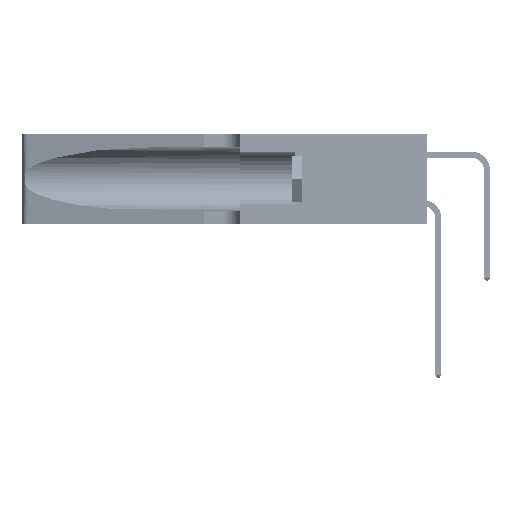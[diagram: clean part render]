
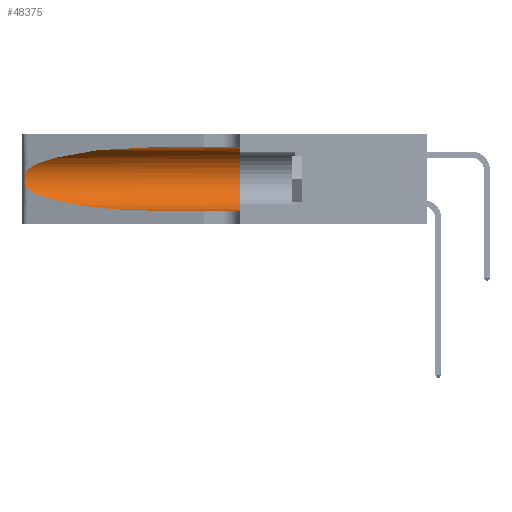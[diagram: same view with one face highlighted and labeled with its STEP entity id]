
A CAD part, left-side view. The second image highlights one B-rep face of the part: STEP entity #48375.
In plain terms, the highlighted cylindrical face has radius 3.308 mm (diameter 6.617 mm), a partial arc.
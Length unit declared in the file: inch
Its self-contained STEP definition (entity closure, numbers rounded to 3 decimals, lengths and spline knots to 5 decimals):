
#54 = ORIENTED_EDGE ( 'NONE', *, *, #10512, .F. ) ;
#1096 = DIRECTION ( 'NONE',  ( 0., 0., 1. ) ) ;
#1575 = CYLINDRICAL_SURFACE ( 'NONE', #9185, 0.13025 ) ;
#2774 = FACE_OUTER_BOUND ( 'NONE', #11011, .T. ) ;
#3232 = DIRECTION ( 'NONE',  ( 0., 0., -1. ) ) ;
#3896 = EDGE_CURVE ( 'NONE', #20273, #45783, #6165, .T. ) ;
#4743 = CARTESIAN_POINT ( 'NONE',  ( 0.25487, 1.22718, 0.14631 ) ) ;
#5531 = VERTEX_POINT ( 'NONE', #31249 ) ;
#5958 = CARTESIAN_POINT ( 'NONE',  ( 0.25787, 1.23484, 0.2124 ) ) ;
#6165 = LINE ( 'NONE', #10392, #45437 ) ;
#8508 = CARTESIAN_POINT ( 'NONE',  ( 0.25487, 1.22718, 0.22369 ) ) ;
#8658 = CARTESIAN_POINT ( 'NONE',  ( 0.2373, 1.15595, 0.08982 ) ) ;
#9185 = AXIS2_PLACEMENT_3D ( 'NONE', #18717, #41415, #3232 ) ;
#9362 = EDGE_CURVE ( 'NONE', #5531, #28183, #43815, .T. ) ;
#9848 = CARTESIAN_POINT ( 'NONE',  ( 0.26018, 1.23835, 0.19895 ) ) ;
#10392 = CARTESIAN_POINT ( 'NONE',  ( 0.1305, 1.61858, 0.05475 ) ) ;
#10512 = EDGE_CURVE ( 'NONE', #43008, #35788, #24158, .T. ) ;
#11011 = EDGE_LOOP ( 'NONE', ( #44678, #37558, #48552, #19919, #36884, #54 ) ) ;
#12550 = CARTESIAN_POINT ( 'NONE',  ( 0.1305, 0.72297, 0.05475 ) ) ;
#12875 = VECTOR ( 'NONE', #21083, 39.37008 ) ;
#13599 = CARTESIAN_POINT ( 'NONE',  ( 0.1305, 1.61858, 0.31525 ) ) ;
#13711 = CARTESIAN_POINT ( 'NONE',  ( 0.26075, 1.23896, 0.178 ) ) ;
#15723 = CIRCLE ( 'NONE', #29706, 0.13025 ) ;
#17556 = CARTESIAN_POINT ( 'NONE',  ( 0.25856, 1.23593, 0.16098 ) ) ;
#18717 = CARTESIAN_POINT ( 'NONE',  ( 0.1305, 1.61858, 0.185 ) ) ;
#19871 = CARTESIAN_POINT ( 'NONE',  ( 0.18966, 0.96281, 0.31525 ) ) ;
#19919 = ORIENTED_EDGE ( 'NONE', *, *, #3896, .T. ) ;
#20273 = VERTEX_POINT ( 'NONE', #47806 ) ;
#21083 = DIRECTION ( 'NONE',  ( 0., -1., 0. ) ) ;
#21197 = CARTESIAN_POINT ( 'NONE',  ( 0.25555, 1.22994, 0.2215 ) ) ;
#21355 = CARTESIAN_POINT ( 'NONE',  ( 0.25639, 1.23186, 0.15144 ) ) ;
#21872 = DIRECTION ( 'NONE',  ( 0., -1., 0. ) ) ;
#23685 = CARTESIAN_POINT ( 'NONE',  ( 0.1305, 0.72297, 0.31525 ) ) ;
#24044 = DIRECTION ( 'NONE',  ( 0., 1., 0. ) ) ;
#24158 = LINE ( 'NONE', #13599, #12875 ) ;
#25163 = CARTESIAN_POINT ( 'NONE',  ( 0.25487, 1.22718, 0.14631 ) ) ;
#26105 = CARTESIAN_POINT ( 'NONE',  ( 0.1305, 0.35, 0.05475 ) ) ;
#26762 = CARTESIAN_POINT ( 'NONE',  ( 0.1305, 0.35, 0.31525 ) ) ;
#27754 =( BOUNDED_CURVE ( )  B_SPLINE_CURVE ( 3, ( #23685, #19871, #31350, #8508 ),
 .UNSPECIFIED., .F., .F. ) 
 B_SPLINE_CURVE_WITH_KNOTS ( ( 4, 4 ),
 ( 1.5708, 2.84003 ),
 .UNSPECIFIED. ) 
 CURVE ( )  GEOMETRIC_REPRESENTATION_ITEM ( )  RATIONAL_B_SPLINE_CURVE ( ( 1., 0.87, 0.87, 1. ) ) 
 REPRESENTATION_ITEM ( '' )  );
#28183 = VERTEX_POINT ( 'NONE', #39303 ) ;
#28840 = CARTESIAN_POINT ( 'NONE',  ( 0.25639, 1.23184, 0.21858 ) ) ;
#29706 = AXIS2_PLACEMENT_3D ( 'NONE', #46726, #24044, #1096 ) ;
#31249 = CARTESIAN_POINT ( 'NONE',  ( 0.25487, 1.22718, 0.22369 ) ) ;
#31350 = CARTESIAN_POINT ( 'NONE',  ( 0.2373, 1.15595, 0.28018 ) ) ;
#32024 = EDGE_CURVE ( 'NONE', #35788, #45783, #15723, .T. ) ;
#32645 = CARTESIAN_POINT ( 'NONE',  ( 0.25854, 1.2359, 0.20912 ) ) ;
#35276 = CARTESIAN_POINT ( 'NONE',  ( 0.18966, 0.96281, 0.05475 ) ) ;
#35788 = VERTEX_POINT ( 'NONE', #26762 ) ;
#36444 = CARTESIAN_POINT ( 'NONE',  ( 0.26075, 1.23896, 0.19203 ) ) ;
#36884 = ORIENTED_EDGE ( 'NONE', *, *, #32024, .F. ) ;
#37143 = EDGE_CURVE ( 'NONE', #28183, #20273, #45331, .T. ) ;
#37558 = ORIENTED_EDGE ( 'NONE', *, *, #9362, .T. ) ;
#39303 = CARTESIAN_POINT ( 'NONE',  ( 0.25487, 1.22718, 0.14631 ) ) ;
#40268 = CARTESIAN_POINT ( 'NONE',  ( 0.26017, 1.23833, 0.17102 ) ) ;
#41415 = DIRECTION ( 'NONE',  ( 0., -1., 0. ) ) ;
#41862 = CARTESIAN_POINT ( 'NONE',  ( 0.1305, 0.72297, 0.31525 ) ) ;
#42454 = EDGE_CURVE ( 'NONE', #43008, #5531, #27754, .T. ) ;
#43008 = VERTEX_POINT ( 'NONE', #41862 ) ;
#43815 = B_SPLINE_CURVE_WITH_KNOTS ( 'NONE', 3,
 ( #47676, #21197, #28840, #5958, #32645, #9848, #36444, #13711, #40268, #17556, #44053, #21355, #47841, #25163 ),
 .UNSPECIFIED., .F., .F.,
 ( 4, 2, 2, 2, 2, 2, 4 ),
 ( 0., 0.00027, 0.00053, 0.00107, 0.0016, 0.00187, 0.00214 ),
 .UNSPECIFIED. ) ;
#44053 = CARTESIAN_POINT ( 'NONE',  ( 0.25789, 1.23486, 0.15765 ) ) ;
#44678 = ORIENTED_EDGE ( 'NONE', *, *, #42454, .T. ) ;
#45331 =( BOUNDED_CURVE ( )  B_SPLINE_CURVE ( 3, ( #4743, #8658, #35276, #12550 ),
 .UNSPECIFIED., .F., .F. ) 
 B_SPLINE_CURVE_WITH_KNOTS ( ( 4, 4 ),
 ( 3.44316, 4.71239 ),
 .UNSPECIFIED. ) 
 CURVE ( )  GEOMETRIC_REPRESENTATION_ITEM ( )  RATIONAL_B_SPLINE_CURVE ( ( 1., 0.87, 0.87, 1. ) ) 
 REPRESENTATION_ITEM ( '' )  );
#45437 = VECTOR ( 'NONE', #21872, 39.37008 ) ;
#45783 = VERTEX_POINT ( 'NONE', #26105 ) ;
#46726 = CARTESIAN_POINT ( 'NONE',  ( 0.1305, 0.35, 0.185 ) ) ;
#47676 = CARTESIAN_POINT ( 'NONE',  ( 0.25487, 1.22718, 0.22369 ) ) ;
#47806 = CARTESIAN_POINT ( 'NONE',  ( 0.1305, 0.72297, 0.05475 ) ) ;
#47841 = CARTESIAN_POINT ( 'NONE',  ( 0.25555, 1.22993, 0.14849 ) ) ;
#48375 = ADVANCED_FACE ( 'NONE', ( #2774 ), #1575, .F. ) ;
#48552 = ORIENTED_EDGE ( 'NONE', *, *, #37143, .T. ) ;
